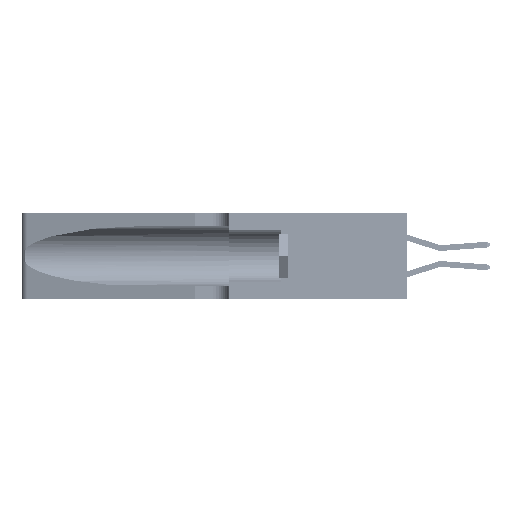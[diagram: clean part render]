
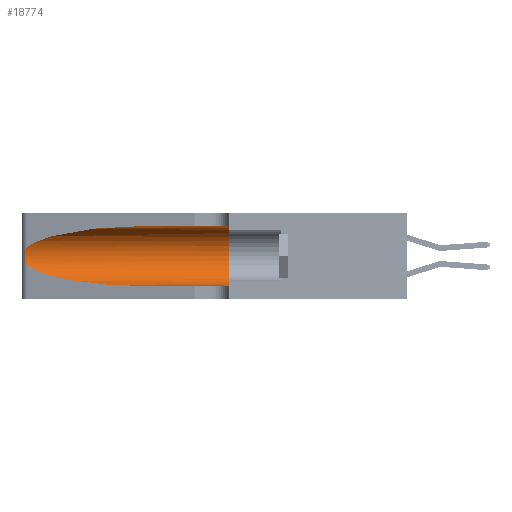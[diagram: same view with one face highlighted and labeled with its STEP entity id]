
A CAD part, left-side view. The second image highlights one B-rep face of the part: STEP entity #18774.
In plain terms, the highlighted cylindrical face has radius 3.308 mm (diameter 6.617 mm), a partial arc.
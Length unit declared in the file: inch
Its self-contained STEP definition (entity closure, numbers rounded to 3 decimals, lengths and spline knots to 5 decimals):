
#2017 = VECTOR ( 'NONE', #5043, 39.37008 ) ;
#2253 = DIRECTION ( 'NONE',  ( 0., 0., -1. ) ) ;
#4895 = CARTESIAN_POINT ( 'NONE',  ( 0.1305, 0.72297, 0.05475 ) ) ;
#5043 = DIRECTION ( 'NONE',  ( 0., -1., 0. ) ) ;
#5870 = CARTESIAN_POINT ( 'NONE',  ( 0.1305, 0.72297, 0.05475 ) ) ;
#6124 = CYLINDRICAL_SURFACE ( 'NONE', #39043, 0.13025 ) ;
#6270 = CARTESIAN_POINT ( 'NONE',  ( 0.1305, 1.61858, 0.185 ) ) ;
#6627 = CARTESIAN_POINT ( 'NONE',  ( 0.26075, 1.23896, 0.19203 ) ) ;
#6637 = CARTESIAN_POINT ( 'NONE',  ( 0.1305, 0.72297, 0.31525 ) ) ;
#6793 = CARTESIAN_POINT ( 'NONE',  ( 0.25639, 1.23184, 0.21858 ) ) ;
#7121 = CARTESIAN_POINT ( 'NONE',  ( 0.25789, 1.23486, 0.15765 ) ) ;
#7978 = EDGE_LOOP ( 'NONE', ( #20623, #43211, #8005, #39302, #22680, #40421 ) ) ;
#7984 = DIRECTION ( 'NONE',  ( 0., 1., 0. ) ) ;
#8005 = ORIENTED_EDGE ( 'NONE', *, *, #12583, .T. ) ;
#9926 = VERTEX_POINT ( 'NONE', #6637 ) ;
#10256 = VERTEX_POINT ( 'NONE', #16327 ) ;
#10284 = DIRECTION ( 'NONE',  ( 0., -1., 0. ) ) ;
#10793 = CARTESIAN_POINT ( 'NONE',  ( 0.26075, 1.23896, 0.178 ) ) ;
#11435 = CIRCLE ( 'NONE', #14220, 0.13025 ) ;
#12583 = EDGE_CURVE ( 'NONE', #10256, #23196, #16800, .T. ) ;
#14220 = AXIS2_PLACEMENT_3D ( 'NONE', #31250, #7984, #46231 ) ;
#14328 = CARTESIAN_POINT ( 'NONE',  ( 0.25639, 1.23186, 0.15144 ) ) ;
#14498 = CARTESIAN_POINT ( 'NONE',  ( 0.25854, 1.2359, 0.20912 ) ) ;
#14529 = FACE_OUTER_BOUND ( 'NONE', #7978, .T. ) ;
#15754 = CARTESIAN_POINT ( 'NONE',  ( 0.1305, 1.61858, 0.05475 ) ) ;
#15884 =( BOUNDED_CURVE ( )  B_SPLINE_CURVE ( 3, ( #18098, #33641, #41372, #37667 ),
 .UNSPECIFIED., .F., .T. ) 
 B_SPLINE_CURVE_WITH_KNOTS ( ( 4, 4 ),
 ( 1.5708, 2.84003 ),
 .UNSPECIFIED. ) 
 CURVE ( )  GEOMETRIC_REPRESENTATION_ITEM ( )  RATIONAL_B_SPLINE_CURVE ( ( 1., 0.87, 0.87, 1. ) ) 
 REPRESENTATION_ITEM ( '' )  );
#16128 = CARTESIAN_POINT ( 'NONE',  ( 0.18966, 0.96281, 0.05475 ) ) ;
#16327 = CARTESIAN_POINT ( 'NONE',  ( 0.25487, 1.22718, 0.14631 ) ) ;
#16800 =( BOUNDED_CURVE ( )  B_SPLINE_CURVE ( 3, ( #46826, #46665, #16128, #4895 ),
 .UNSPECIFIED., .F., .F. ) 
 B_SPLINE_CURVE_WITH_KNOTS ( ( 4, 4 ),
 ( 3.44316, 4.71239 ),
 .UNSPECIFIED. ) 
 CURVE ( )  GEOMETRIC_REPRESENTATION_ITEM ( )  RATIONAL_B_SPLINE_CURVE ( ( 1., 0.87, 0.87, 1. ) ) 
 REPRESENTATION_ITEM ( '' )  );
#18098 = CARTESIAN_POINT ( 'NONE',  ( 0.1305, 0.72297, 0.31525 ) ) ;
#18429 = CARTESIAN_POINT ( 'NONE',  ( 0.1305, 0.35, 0.31525 ) ) ;
#18532 = CARTESIAN_POINT ( 'NONE',  ( 0.25856, 1.23593, 0.16098 ) ) ;
#18774 = ADVANCED_FACE ( 'NONE', ( #14529 ), #6124, .F. ) ;
#20455 = CARTESIAN_POINT ( 'NONE',  ( 0.1305, 1.61858, 0.31525 ) ) ;
#20623 = ORIENTED_EDGE ( 'NONE', *, *, #27607, .T. ) ;
#21974 = EDGE_CURVE ( 'NONE', #32012, #10256, #22617, .T. ) ;
#22201 = CARTESIAN_POINT ( 'NONE',  ( 0.25555, 1.22994, 0.2215 ) ) ;
#22617 = B_SPLINE_CURVE_WITH_KNOTS ( 'NONE', 3,
 ( #29715, #22201, #6793, #37763, #14498, #33571, #6627, #10793, #49060, #18532, #7121, #14328, #26188, #37426 ),
 .UNSPECIFIED., .F., .F.,
 ( 4, 2, 2, 2, 2, 2, 4 ),
 ( 0., 0.00027, 0.00053, 0.00107, 0.0016, 0.00187, 0.00214 ),
 .UNSPECIFIED. ) ;
#22680 = ORIENTED_EDGE ( 'NONE', *, *, #24720, .F. ) ;
#23137 = VERTEX_POINT ( 'NONE', #47969 ) ;
#23196 = VERTEX_POINT ( 'NONE', #5870 ) ;
#24720 = EDGE_CURVE ( 'NONE', #32524, #23137, #11435, .T. ) ;
#26188 = CARTESIAN_POINT ( 'NONE',  ( 0.25555, 1.22993, 0.14849 ) ) ;
#26803 = CARTESIAN_POINT ( 'NONE',  ( 0.25487, 1.22718, 0.22369 ) ) ;
#27607 = EDGE_CURVE ( 'NONE', #9926, #32012, #15884, .T. ) ;
#29715 = CARTESIAN_POINT ( 'NONE',  ( 0.25487, 1.22718, 0.22369 ) ) ;
#31250 = CARTESIAN_POINT ( 'NONE',  ( 0.1305, 0.35, 0.185 ) ) ;
#32012 = VERTEX_POINT ( 'NONE', #26803 ) ;
#32524 = VERTEX_POINT ( 'NONE', #18429 ) ;
#33571 = CARTESIAN_POINT ( 'NONE',  ( 0.26018, 1.23835, 0.19895 ) ) ;
#33641 = CARTESIAN_POINT ( 'NONE',  ( 0.18966, 0.96281, 0.31525 ) ) ;
#34957 = LINE ( 'NONE', #20455, #2017 ) ;
#35463 = EDGE_CURVE ( 'NONE', #23196, #23137, #36450, .T. ) ;
#36450 = LINE ( 'NONE', #15754, #39496 ) ;
#37426 = CARTESIAN_POINT ( 'NONE',  ( 0.25487, 1.22718, 0.14631 ) ) ;
#37667 = CARTESIAN_POINT ( 'NONE',  ( 0.25487, 1.22718, 0.22369 ) ) ;
#37763 = CARTESIAN_POINT ( 'NONE',  ( 0.25787, 1.23484, 0.2124 ) ) ;
#38381 = EDGE_CURVE ( 'NONE', #9926, #32524, #34957, .T. ) ;
#39043 = AXIS2_PLACEMENT_3D ( 'NONE', #6270, #10284, #2253 ) ;
#39302 = ORIENTED_EDGE ( 'NONE', *, *, #35463, .T. ) ;
#39496 = VECTOR ( 'NONE', #42584, 39.37008 ) ;
#40421 = ORIENTED_EDGE ( 'NONE', *, *, #38381, .F. ) ;
#41372 = CARTESIAN_POINT ( 'NONE',  ( 0.2373, 1.15595, 0.28018 ) ) ;
#42584 = DIRECTION ( 'NONE',  ( 0., -1., 0. ) ) ;
#43211 = ORIENTED_EDGE ( 'NONE', *, *, #21974, .T. ) ;
#46231 = DIRECTION ( 'NONE',  ( 0., 0., 1. ) ) ;
#46665 = CARTESIAN_POINT ( 'NONE',  ( 0.2373, 1.15595, 0.08982 ) ) ;
#46826 = CARTESIAN_POINT ( 'NONE',  ( 0.25487, 1.22718, 0.14631 ) ) ;
#47969 = CARTESIAN_POINT ( 'NONE',  ( 0.1305, 0.35, 0.05475 ) ) ;
#49060 = CARTESIAN_POINT ( 'NONE',  ( 0.26017, 1.23833, 0.17102 ) ) ;
